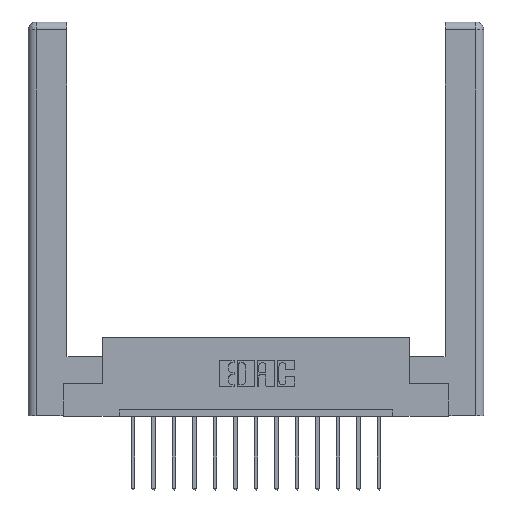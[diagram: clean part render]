
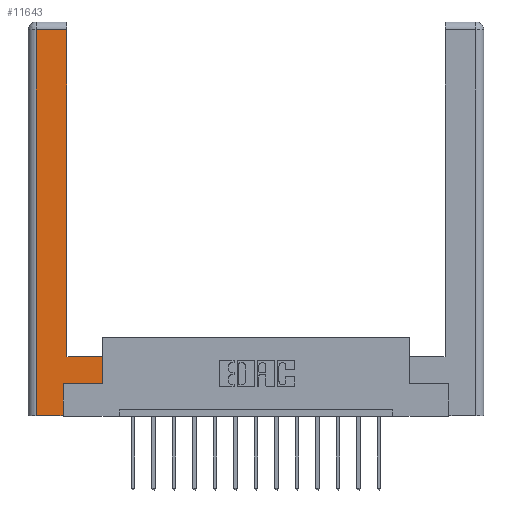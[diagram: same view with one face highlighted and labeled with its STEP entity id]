
A CAD part, top view. The second image highlights one B-rep face of the part: STEP entity #11643.
In plain terms, the highlighted planar face has unit normal (0, 0, 1).
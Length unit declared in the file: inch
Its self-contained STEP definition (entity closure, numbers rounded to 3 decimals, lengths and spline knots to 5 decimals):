
#13 = LINE ( 'NONE', #972, #1150 ) ;
#763 = VERTEX_POINT ( 'NONE', #2979 ) ;
#972 = CARTESIAN_POINT ( 'NONE',  ( 0.295, 0.45, 0. ) ) ;
#1150 = VECTOR ( 'NONE', #3346, 39.37008 ) ;
#1400 = EDGE_CURVE ( 'NONE', #9349, #763, #10778, .T. ) ;
#1742 = CARTESIAN_POINT ( 'NONE',  ( 0.265, 0., 0. ) ) ;
#1784 = ORIENTED_EDGE ( 'NONE', *, *, #5140, .T. ) ;
#2534 = ORIENTED_EDGE ( 'NONE', *, *, #12673, .T. ) ;
#2979 = CARTESIAN_POINT ( 'NONE',  ( 0.0615, 2.94, 0. ) ) ;
#3055 = LINE ( 'NONE', #15250, #11188 ) ;
#3153 = CARTESIAN_POINT ( 'NONE',  ( 0.0615, 2.94, 0. ) ) ;
#3346 = DIRECTION ( 'NONE',  ( -1., 0., 0. ) ) ;
#3440 = ORIENTED_EDGE ( 'NONE', *, *, #8213, .T. ) ;
#3513 = LINE ( 'NONE', #8731, #4866 ) ;
#3690 = AXIS2_PLACEMENT_3D ( 'NONE', #4473, #8106, #15732 ) ;
#3771 = CARTESIAN_POINT ( 'NONE',  ( 0.265, 0.245, 0. ) ) ;
#3968 = LINE ( 'NONE', #11344, #9225 ) ;
#4473 = CARTESIAN_POINT ( 'NONE',  ( 0., 0., 0. ) ) ;
#4866 = VECTOR ( 'NONE', #6431, 39.37008 ) ;
#5016 = DIRECTION ( 'NONE',  ( 0., 1., 0. ) ) ;
#5036 = FACE_OUTER_BOUND ( 'NONE', #12207, .T. ) ;
#5140 = EDGE_CURVE ( 'NONE', #13102, #10513, #8879, .T. ) ;
#5502 = DIRECTION ( 'NONE',  ( -1., 0., 0. ) ) ;
#5708 = PLANE ( 'NONE',  #3690 ) ;
#6028 = ORIENTED_EDGE ( 'NONE', *, *, #13630, .T. ) ;
#6205 = CARTESIAN_POINT ( 'NONE',  ( 0.565, 0.245, 0. ) ) ;
#6431 = DIRECTION ( 'NONE',  ( 1., 0., 0. ) ) ;
#7403 = VERTEX_POINT ( 'NONE', #6205 ) ;
#7536 = DIRECTION ( 'NONE',  ( 0., 1., 0. ) ) ;
#8106 = DIRECTION ( 'NONE',  ( 0., 0., -1. ) ) ;
#8213 = EDGE_CURVE ( 'NONE', #13799, #13102, #3513, .T. ) ;
#8305 = VECTOR ( 'NONE', #11363, 39.37008 ) ;
#8731 = CARTESIAN_POINT ( 'NONE',  ( 0.265, 0., 0. ) ) ;
#8768 = CARTESIAN_POINT ( 'NONE',  ( 0.565, 0.45, 0. ) ) ;
#8879 = LINE ( 'NONE', #3771, #11193 ) ;
#9225 = VECTOR ( 'NONE', #9927, 39.37008 ) ;
#9349 = VERTEX_POINT ( 'NONE', #9585 ) ;
#9446 = VERTEX_POINT ( 'NONE', #13196 ) ;
#9581 = EDGE_CURVE ( 'NONE', #9446, #9349, #3968, .T. ) ;
#9585 = CARTESIAN_POINT ( 'NONE',  ( 0.295, 2.94, 0. ) ) ;
#9927 = DIRECTION ( 'NONE',  ( 0., 1., 0. ) ) ;
#10342 = DIRECTION ( 'NONE',  ( 0., -1., 0. ) ) ;
#10513 = VERTEX_POINT ( 'NONE', #14339 ) ;
#10778 = LINE ( 'NONE', #3153, #15054 ) ;
#11188 = VECTOR ( 'NONE', #10342, 39.37008 ) ;
#11193 = VECTOR ( 'NONE', #5016, 39.37008 ) ;
#11263 = CARTESIAN_POINT ( 'NONE',  ( 0.565, 0.245, 0. ) ) ;
#11344 = CARTESIAN_POINT ( 'NONE',  ( 0.295, 3., 0. ) ) ;
#11363 = DIRECTION ( 'NONE',  ( 1., 0., 0. ) ) ;
#11643 = ADVANCED_FACE ( 'NONE', ( #5036 ), #5708, .F. ) ;
#11913 = LINE ( 'NONE', #8768, #14834 ) ;
#12207 = EDGE_LOOP ( 'NONE', ( #12651, #13700, #2534, #3440, #1784, #15334, #6028, #14764 ) ) ;
#12275 = EDGE_CURVE ( 'NONE', #10513, #7403, #12564, .T. ) ;
#12401 = VERTEX_POINT ( 'NONE', #12430 ) ;
#12430 = CARTESIAN_POINT ( 'NONE',  ( 0.565, 0.45, 0. ) ) ;
#12564 = LINE ( 'NONE', #11263, #8305 ) ;
#12651 = ORIENTED_EDGE ( 'NONE', *, *, #9581, .T. ) ;
#12673 = EDGE_CURVE ( 'NONE', #763, #13799, #3055, .T. ) ;
#12819 = CARTESIAN_POINT ( 'NONE',  ( 0.0615, 0., 0. ) ) ;
#13102 = VERTEX_POINT ( 'NONE', #1742 ) ;
#13196 = CARTESIAN_POINT ( 'NONE',  ( 0.295, 0.45, 0. ) ) ;
#13630 = EDGE_CURVE ( 'NONE', #7403, #12401, #11913, .T. ) ;
#13700 = ORIENTED_EDGE ( 'NONE', *, *, #1400, .T. ) ;
#13799 = VERTEX_POINT ( 'NONE', #12819 ) ;
#14339 = CARTESIAN_POINT ( 'NONE',  ( 0.265, 0.245, 0. ) ) ;
#14764 = ORIENTED_EDGE ( 'NONE', *, *, #14959, .T. ) ;
#14834 = VECTOR ( 'NONE', #7536, 39.37008 ) ;
#14959 = EDGE_CURVE ( 'NONE', #12401, #9446, #13, .T. ) ;
#15054 = VECTOR ( 'NONE', #5502, 39.37008 ) ;
#15250 = CARTESIAN_POINT ( 'NONE',  ( 0.0615, 0., 0. ) ) ;
#15334 = ORIENTED_EDGE ( 'NONE', *, *, #12275, .T. ) ;
#15732 = DIRECTION ( 'NONE',  ( -1., 0., 0. ) ) ;
